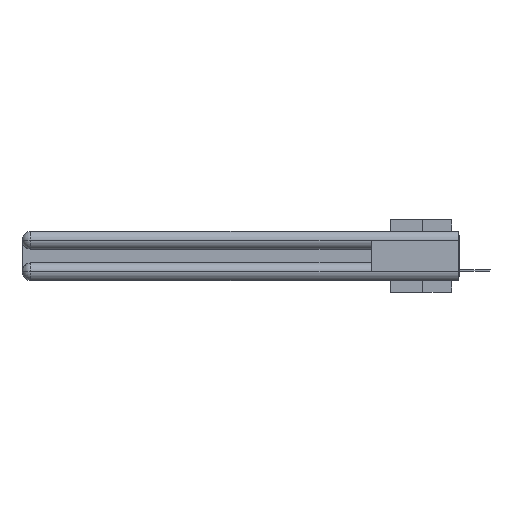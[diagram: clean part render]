
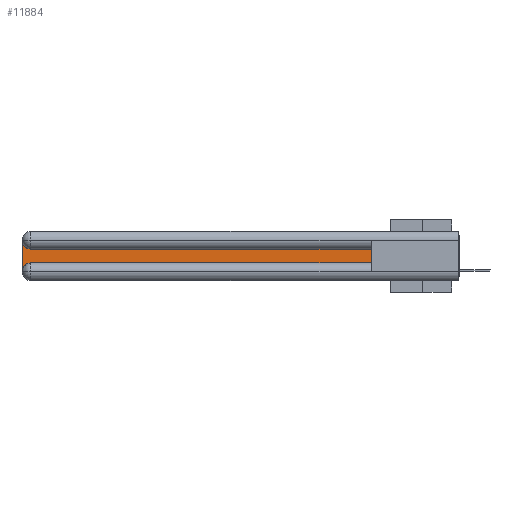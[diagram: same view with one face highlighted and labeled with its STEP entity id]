
A CAD part, left-side view. The second image highlights one B-rep face of the part: STEP entity #11884.
In plain terms, the highlighted planar face has unit normal (-1, 0, 0).
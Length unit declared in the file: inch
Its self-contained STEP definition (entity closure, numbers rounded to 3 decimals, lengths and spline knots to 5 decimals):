
#1048 = CARTESIAN_POINT ( 'NONE',  ( 0.075, 0.6, -0.2175 ) ) ;
#4149 = ORIENTED_EDGE ( 'NONE', *, *, #26683, .T. ) ;
#6464 = DIRECTION ( 'NONE',  ( 0., 0., -1. ) ) ;
#7301 = CARTESIAN_POINT ( 'NONE',  ( 0.075, 0.6, -0.2175 ) ) ;
#7380 = ORIENTED_EDGE ( 'NONE', *, *, #28822, .T. ) ;
#7391 = DIRECTION ( 'NONE',  ( 1., 0., 0. ) ) ;
#7605 = EDGE_CURVE ( 'NONE', #28910, #17845, #15990, .T. ) ;
#7893 = DIRECTION ( 'NONE',  ( 0., 0., -1. ) ) ;
#9010 = DIRECTION ( 'NONE',  ( 1., 0., 0. ) ) ;
#9080 = LINE ( 'NONE', #15167, #34629 ) ;
#10420 = DIRECTION ( 'NONE',  ( 0., 1., 0. ) ) ;
#11542 = CARTESIAN_POINT ( 'NONE',  ( 0.075, 3., -0.1225 ) ) ;
#11884 = ADVANCED_FACE ( 'NONE', ( #34116 ), #26023, .F. ) ;
#12261 = DIRECTION ( 'NONE',  ( 0., 0., 1. ) ) ;
#12998 = DIRECTION ( 'NONE',  ( 0., 0., -1. ) ) ;
#13337 = AXIS2_PLACEMENT_3D ( 'NONE', #27887, #7391, #12998 ) ;
#13339 = VECTOR ( 'NONE', #10420, 39.37008 ) ;
#15046 = CIRCLE ( 'NONE', #13337, 0.06 ) ;
#15167 = CARTESIAN_POINT ( 'NONE',  ( 0.075, 0.6, -0.2175 ) ) ;
#15990 = LINE ( 'NONE', #22150, #35755 ) ;
#16002 = CARTESIAN_POINT ( 'NONE',  ( 0.075, 0.6, -0.1225 ) ) ;
#16857 = CARTESIAN_POINT ( 'NONE',  ( 0.075, 2.94, -0.2175 ) ) ;
#17018 = VERTEX_POINT ( 'NONE', #30512 ) ;
#17753 = EDGE_CURVE ( 'NONE', #17845, #22477, #31033, .T. ) ;
#17845 = VERTEX_POINT ( 'NONE', #35657 ) ;
#18340 = DIRECTION ( 'NONE',  ( 1., 0., 0. ) ) ;
#18535 = ORIENTED_EDGE ( 'NONE', *, *, #17753, .T. ) ;
#19034 = ORIENTED_EDGE ( 'NONE', *, *, #26908, .T. ) ;
#21808 = VECTOR ( 'NONE', #34895, 39.37008 ) ;
#22123 = VERTEX_POINT ( 'NONE', #7301 ) ;
#22150 = CARTESIAN_POINT ( 'NONE',  ( 0.075, 3., -0.2175 ) ) ;
#22477 = VERTEX_POINT ( 'NONE', #16857 ) ;
#23395 = DIRECTION ( 'NONE',  ( 0., 0., -1. ) ) ;
#23853 = CARTESIAN_POINT ( 'NONE',  ( 0.075, 2.94, -0.2775 ) ) ;
#25874 = AXIS2_PLACEMENT_3D ( 'NONE', #11542, #9010, #23395 ) ;
#26023 = PLANE ( 'NONE',  #25874 ) ;
#26683 = EDGE_CURVE ( 'NONE', #17018, #28968, #34793, .T. ) ;
#26742 = EDGE_CURVE ( 'NONE', #28968, #28910, #15046, .T. ) ;
#26908 = EDGE_CURVE ( 'NONE', #22477, #22123, #30306, .T. ) ;
#27887 = CARTESIAN_POINT ( 'NONE',  ( 0.075, 2.94, -0.0625 ) ) ;
#28822 = EDGE_CURVE ( 'NONE', #22123, #17018, #9080, .T. ) ;
#28910 = VERTEX_POINT ( 'NONE', #29902 ) ;
#28968 = VERTEX_POINT ( 'NONE', #35579 ) ;
#29902 = CARTESIAN_POINT ( 'NONE',  ( 0.075, 3., -0.0625 ) ) ;
#30082 = ORIENTED_EDGE ( 'NONE', *, *, #26742, .T. ) ;
#30306 = LINE ( 'NONE', #1048, #21808 ) ;
#30512 = CARTESIAN_POINT ( 'NONE',  ( 0.075, 0.6, -0.1225 ) ) ;
#31033 = CIRCLE ( 'NONE', #32473, 0.06 ) ;
#32473 = AXIS2_PLACEMENT_3D ( 'NONE', #23853, #18340, #6464 ) ;
#33152 = ORIENTED_EDGE ( 'NONE', *, *, #7605, .T. ) ;
#33923 = EDGE_LOOP ( 'NONE', ( #4149, #30082, #33152, #18535, #19034, #7380 ) ) ;
#34116 = FACE_OUTER_BOUND ( 'NONE', #33923, .T. ) ;
#34629 = VECTOR ( 'NONE', #12261, 39.37008 ) ;
#34793 = LINE ( 'NONE', #16002, #13339 ) ;
#34895 = DIRECTION ( 'NONE',  ( 0., -1., 0. ) ) ;
#35579 = CARTESIAN_POINT ( 'NONE',  ( 0.075, 2.94, -0.1225 ) ) ;
#35657 = CARTESIAN_POINT ( 'NONE',  ( 0.075, 3., -0.2775 ) ) ;
#35755 = VECTOR ( 'NONE', #7893, 39.37008 ) ;
